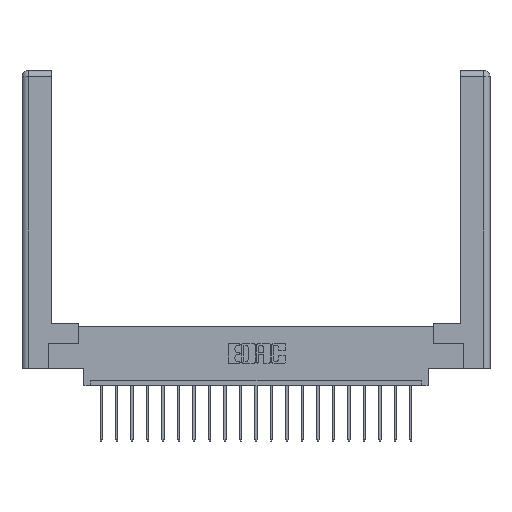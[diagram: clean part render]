
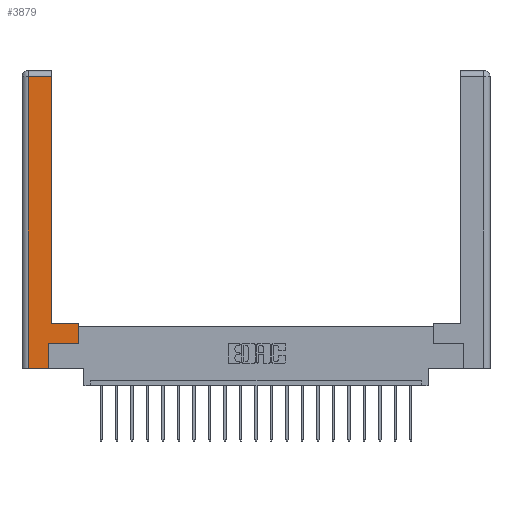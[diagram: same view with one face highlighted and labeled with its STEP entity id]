
A CAD part, top view. The second image highlights one B-rep face of the part: STEP entity #3879.
In plain terms, the highlighted planar face has unit normal (0, 0, 1).
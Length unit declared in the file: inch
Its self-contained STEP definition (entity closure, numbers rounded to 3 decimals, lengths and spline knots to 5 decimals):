
#96 = CARTESIAN_POINT ( 'NONE',  ( 0.565, 0.245, 0. ) ) ;
#499 = EDGE_CURVE ( 'NONE', #12346, #2354, #11675, .T. ) ;
#681 = EDGE_CURVE ( 'NONE', #1805, #12346, #16519, .T. ) ;
#958 = CARTESIAN_POINT ( 'NONE',  ( 0.565, 0.45, 0. ) ) ;
#1755 = LINE ( 'NONE', #19513, #18865 ) ;
#1805 = VERTEX_POINT ( 'NONE', #5736 ) ;
#2354 = VERTEX_POINT ( 'NONE', #958 ) ;
#2577 = ORIENTED_EDGE ( 'NONE', *, *, #681, .T. ) ;
#2671 = EDGE_CURVE ( 'NONE', #10674, #16125, #15557, .T. ) ;
#3465 = VERTEX_POINT ( 'NONE', #19855 ) ;
#3858 = DIRECTION ( 'NONE',  ( 0., 1., 0. ) ) ;
#3879 = ADVANCED_FACE ( 'NONE', ( #19395 ), #11237, .F. ) ;
#5614 = ORIENTED_EDGE ( 'NONE', *, *, #18153, .T. ) ;
#5625 = CARTESIAN_POINT ( 'NONE',  ( 0.295, 0.45, 0. ) ) ;
#5733 = DIRECTION ( 'NONE',  ( -1., 0., 0. ) ) ;
#5736 = CARTESIAN_POINT ( 'NONE',  ( 0.265, 0.245, 0. ) ) ;
#6527 = DIRECTION ( 'NONE',  ( -1., 0., 0. ) ) ;
#6532 = VECTOR ( 'NONE', #3858, 39.37008 ) ;
#6612 = EDGE_LOOP ( 'NONE', ( #20917, #10469, #11931, #13228, #10614, #2577, #19493, #5614 ) ) ;
#7180 = LINE ( 'NONE', #11431, #13307 ) ;
#7338 = EDGE_CURVE ( 'NONE', #17343, #10674, #10522, .T. ) ;
#7799 = AXIS2_PLACEMENT_3D ( 'NONE', #14489, #15154, #15504 ) ;
#8756 = EDGE_CURVE ( 'NONE', #20266, #17343, #11267, .T. ) ;
#8974 = EDGE_CURVE ( 'NONE', #16125, #3465, #16107, .T. ) ;
#9070 = CARTESIAN_POINT ( 'NONE',  ( 0.295, 3., 0. ) ) ;
#9233 = VECTOR ( 'NONE', #5733, 39.37008 ) ;
#9702 = DIRECTION ( 'NONE',  ( 0., 1., 0. ) ) ;
#9968 = EDGE_CURVE ( 'NONE', #3465, #1805, #1755, .T. ) ;
#10469 = ORIENTED_EDGE ( 'NONE', *, *, #7338, .T. ) ;
#10522 = LINE ( 'NONE', #17041, #9233 ) ;
#10614 = ORIENTED_EDGE ( 'NONE', *, *, #9968, .T. ) ;
#10674 = VERTEX_POINT ( 'NONE', #12260 ) ;
#10696 = CARTESIAN_POINT ( 'NONE',  ( 0.0615, 0., 0. ) ) ;
#10749 = VECTOR ( 'NONE', #15808, 39.37008 ) ;
#11237 = PLANE ( 'NONE',  #7799 ) ;
#11267 = LINE ( 'NONE', #9070, #10749 ) ;
#11319 = DIRECTION ( 'NONE',  ( 1., 0., 0. ) ) ;
#11431 = CARTESIAN_POINT ( 'NONE',  ( 0.295, 0.45, 0. ) ) ;
#11508 = DIRECTION ( 'NONE',  ( 1., 0., 0. ) ) ;
#11675 = LINE ( 'NONE', #17936, #6532 ) ;
#11931 = ORIENTED_EDGE ( 'NONE', *, *, #2671, .T. ) ;
#12260 = CARTESIAN_POINT ( 'NONE',  ( 0.0615, 2.94, 0. ) ) ;
#12346 = VERTEX_POINT ( 'NONE', #17451 ) ;
#13162 = VECTOR ( 'NONE', #11508, 39.37008 ) ;
#13228 = ORIENTED_EDGE ( 'NONE', *, *, #8974, .T. ) ;
#13307 = VECTOR ( 'NONE', #6527, 39.37008 ) ;
#14489 = CARTESIAN_POINT ( 'NONE',  ( 0., 0., 0. ) ) ;
#14712 = CARTESIAN_POINT ( 'NONE',  ( 0.265, 0., 0. ) ) ;
#15154 = DIRECTION ( 'NONE',  ( 0., 0., -1. ) ) ;
#15309 = VECTOR ( 'NONE', #20881, 39.37008 ) ;
#15504 = DIRECTION ( 'NONE',  ( -1., 0., 0. ) ) ;
#15557 = LINE ( 'NONE', #10696, #15309 ) ;
#15808 = DIRECTION ( 'NONE',  ( 0., 1., 0. ) ) ;
#16107 = LINE ( 'NONE', #14712, #18670 ) ;
#16125 = VERTEX_POINT ( 'NONE', #19807 ) ;
#16519 = LINE ( 'NONE', #96, #13162 ) ;
#17041 = CARTESIAN_POINT ( 'NONE',  ( 0.0615, 2.94, 0. ) ) ;
#17343 = VERTEX_POINT ( 'NONE', #18087 ) ;
#17451 = CARTESIAN_POINT ( 'NONE',  ( 0.565, 0.245, 0. ) ) ;
#17936 = CARTESIAN_POINT ( 'NONE',  ( 0.565, 0.45, 0. ) ) ;
#18087 = CARTESIAN_POINT ( 'NONE',  ( 0.295, 2.94, 0. ) ) ;
#18153 = EDGE_CURVE ( 'NONE', #2354, #20266, #7180, .T. ) ;
#18670 = VECTOR ( 'NONE', #11319, 39.37008 ) ;
#18865 = VECTOR ( 'NONE', #9702, 39.37008 ) ;
#19395 = FACE_OUTER_BOUND ( 'NONE', #6612, .T. ) ;
#19493 = ORIENTED_EDGE ( 'NONE', *, *, #499, .T. ) ;
#19513 = CARTESIAN_POINT ( 'NONE',  ( 0.265, 0.245, 0. ) ) ;
#19807 = CARTESIAN_POINT ( 'NONE',  ( 0.0615, 0., 0. ) ) ;
#19855 = CARTESIAN_POINT ( 'NONE',  ( 0.265, 0., 0. ) ) ;
#20266 = VERTEX_POINT ( 'NONE', #5625 ) ;
#20881 = DIRECTION ( 'NONE',  ( 0., -1., 0. ) ) ;
#20917 = ORIENTED_EDGE ( 'NONE', *, *, #8756, .T. ) ;
